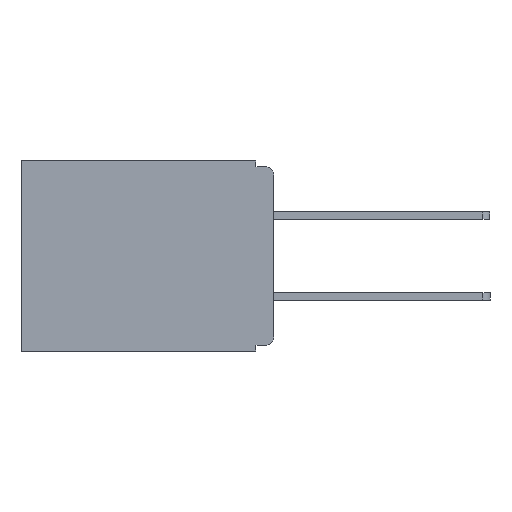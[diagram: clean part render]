
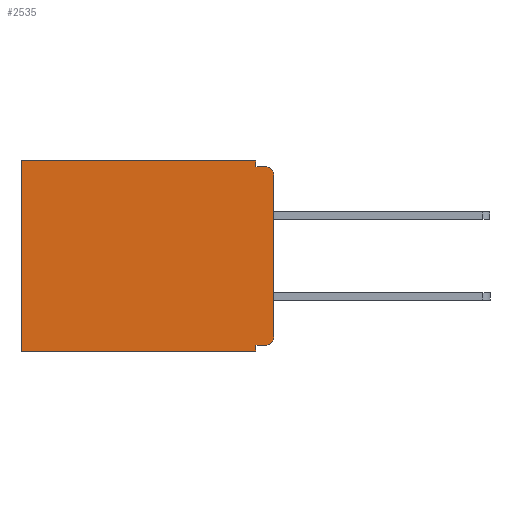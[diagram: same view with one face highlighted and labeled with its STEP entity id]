
A CAD part, left-side view. The second image highlights one B-rep face of the part: STEP entity #2535.
In plain terms, the highlighted planar face has unit normal (-1, 0, 0).
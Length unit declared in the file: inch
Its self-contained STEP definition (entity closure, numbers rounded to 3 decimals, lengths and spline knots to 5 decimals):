
#413 = ORIENTED_EDGE ( 'NONE', *, *, #1137, .T. ) ;
#1073 = DIRECTION ( 'NONE',  ( 1., 0., 0. ) ) ;
#1109 = DIRECTION ( 'NONE',  ( 0., 0., -1. ) ) ;
#1132 = PLANE ( 'NONE',  #11565 ) ;
#1137 = EDGE_CURVE ( 'NONE', #4834, #5431, #10066, .T. ) ;
#1713 = EDGE_CURVE ( 'NONE', #15782, #9134, #15542, .T. ) ;
#1774 = AXIS2_PLACEMENT_3D ( 'NONE', #14150, #14082, #16078 ) ;
#1932 = EDGE_CURVE ( 'NONE', #13408, #7439, #9005, .T. ) ;
#1935 = ORIENTED_EDGE ( 'NONE', *, *, #7380, .F. ) ;
#2269 = FACE_OUTER_BOUND ( 'NONE', #6078, .T. ) ;
#2293 = LINE ( 'NONE', #7403, #15918 ) ;
#2380 = ORIENTED_EDGE ( 'NONE', *, *, #4216, .F. ) ;
#2535 = ADVANCED_FACE ( 'NONE', ( #2269 ), #1132, .F. ) ;
#2682 = CARTESIAN_POINT ( 'NONE',  ( 0.3, 0.031, 0. ) ) ;
#3241 = EDGE_CURVE ( 'NONE', #10888, #13408, #11963, .T. ) ;
#4011 = LINE ( 'NONE', #2682, #7269 ) ;
#4216 = EDGE_CURVE ( 'NONE', #4271, #15782, #4011, .T. ) ;
#4271 = VERTEX_POINT ( 'NONE', #10977 ) ;
#4834 = VERTEX_POINT ( 'NONE', #14305 ) ;
#5072 = EDGE_CURVE ( 'NONE', #9587, #7439, #12307, .T. ) ;
#5298 = VECTOR ( 'NONE', #8970, 39.37008 ) ;
#5418 = VECTOR ( 'NONE', #11537, 39.37008 ) ;
#5431 = VERTEX_POINT ( 'NONE', #10803 ) ;
#5956 = CARTESIAN_POINT ( 'NONE',  ( 0.3, 0.437, -0.33 ) ) ;
#6078 = EDGE_LOOP ( 'NONE', ( #1935, #9300, #16006, #2380, #6184, #10108, #16790, #10494, #13841, #413 ) ) ;
#6184 = ORIENTED_EDGE ( 'NONE', *, *, #15045, .T. ) ;
#6335 = VERTEX_POINT ( 'NONE', #13143 ) ;
#6821 = EDGE_CURVE ( 'NONE', #6335, #9134, #17158, .T. ) ;
#6931 = DIRECTION ( 'NONE',  ( 0., 1., 0. ) ) ;
#6999 = DIRECTION ( 'NONE',  ( 0., 0., -1. ) ) ;
#7269 = VECTOR ( 'NONE', #10260, 39.37008 ) ;
#7380 = EDGE_CURVE ( 'NONE', #6335, #5431, #9245, .T. ) ;
#7403 = CARTESIAN_POINT ( 'NONE',  ( 0.3, 0., -0.32 ) ) ;
#7439 = VERTEX_POINT ( 'NONE', #5956 ) ;
#7558 = DIRECTION ( 'NONE',  ( 0., 0., -1. ) ) ;
#7664 = CARTESIAN_POINT ( 'NONE',  ( 0.3, 0., -0.33 ) ) ;
#7794 = CARTESIAN_POINT ( 'NONE',  ( 0.3, 0.437, -0.33 ) ) ;
#8663 = VECTOR ( 'NONE', #7558, 39.37008 ) ;
#8970 = DIRECTION ( 'NONE',  ( 0., 0., -1. ) ) ;
#9005 = LINE ( 'NONE', #14674, #5418 ) ;
#9134 = VERTEX_POINT ( 'NONE', #9169 ) ;
#9169 = CARTESIAN_POINT ( 'NONE',  ( 0.3, 0.015, -0.01 ) ) ;
#9245 = LINE ( 'NONE', #7664, #8663 ) ;
#9300 = ORIENTED_EDGE ( 'NONE', *, *, #6821, .T. ) ;
#9587 = VERTEX_POINT ( 'NONE', #12559 ) ;
#10066 = CIRCLE ( 'NONE', #1774, 0.015 ) ;
#10108 = ORIENTED_EDGE ( 'NONE', *, *, #5072, .T. ) ;
#10260 = DIRECTION ( 'NONE',  ( 0., 0., -1. ) ) ;
#10327 = EDGE_CURVE ( 'NONE', #4834, #10888, #2293, .T. ) ;
#10494 = ORIENTED_EDGE ( 'NONE', *, *, #3241, .F. ) ;
#10803 = CARTESIAN_POINT ( 'NONE',  ( 0.3, 0., -0.305 ) ) ;
#10888 = VERTEX_POINT ( 'NONE', #16247 ) ;
#10977 = CARTESIAN_POINT ( 'NONE',  ( 0.3, 0.031, 0. ) ) ;
#10994 = AXIS2_PLACEMENT_3D ( 'NONE', #16998, #16992, #16958 ) ;
#11537 = DIRECTION ( 'NONE',  ( 0., 1., 0. ) ) ;
#11551 = VECTOR ( 'NONE', #6999, 39.37008 ) ;
#11565 = AXIS2_PLACEMENT_3D ( 'NONE', #11581, #1073, #1109 ) ;
#11581 = CARTESIAN_POINT ( 'NONE',  ( 0.3, 0., -0.33 ) ) ;
#11963 = LINE ( 'NONE', #17038, #11551 ) ;
#12228 = VECTOR ( 'NONE', #13439, 39.37008 ) ;
#12297 = CARTESIAN_POINT ( 'NONE',  ( 0.3, 0.031, -0.01 ) ) ;
#12307 = LINE ( 'NONE', #7794, #5298 ) ;
#12559 = CARTESIAN_POINT ( 'NONE',  ( 0.3, 0.437, 0. ) ) ;
#13143 = CARTESIAN_POINT ( 'NONE',  ( 0.3, 0., -0.025 ) ) ;
#13408 = VERTEX_POINT ( 'NONE', #16879 ) ;
#13436 = CARTESIAN_POINT ( 'NONE',  ( 0.3, 0., -0.01 ) ) ;
#13439 = DIRECTION ( 'NONE',  ( 0., -1., 0. ) ) ;
#13504 = LINE ( 'NONE', #15857, #15666 ) ;
#13841 = ORIENTED_EDGE ( 'NONE', *, *, #10327, .F. ) ;
#14082 = DIRECTION ( 'NONE',  ( -1., 0., 0. ) ) ;
#14150 = CARTESIAN_POINT ( 'NONE',  ( 0.3, 0.015, -0.305 ) ) ;
#14305 = CARTESIAN_POINT ( 'NONE',  ( 0.3, 0.015, -0.32 ) ) ;
#14674 = CARTESIAN_POINT ( 'NONE',  ( 0.3, 0., -0.33 ) ) ;
#15045 = EDGE_CURVE ( 'NONE', #4271, #9587, #13504, .T. ) ;
#15061 = DIRECTION ( 'NONE',  ( 0., 1., 0. ) ) ;
#15542 = LINE ( 'NONE', #13436, #12228 ) ;
#15666 = VECTOR ( 'NONE', #6931, 39.37008 ) ;
#15782 = VERTEX_POINT ( 'NONE', #12297 ) ;
#15857 = CARTESIAN_POINT ( 'NONE',  ( 0.3, 0., 0. ) ) ;
#15918 = VECTOR ( 'NONE', #15061, 39.37008 ) ;
#16006 = ORIENTED_EDGE ( 'NONE', *, *, #1713, .F. ) ;
#16078 = DIRECTION ( 'NONE',  ( 0., 0., -1. ) ) ;
#16247 = CARTESIAN_POINT ( 'NONE',  ( 0.3, 0.031, -0.32 ) ) ;
#16790 = ORIENTED_EDGE ( 'NONE', *, *, #1932, .F. ) ;
#16879 = CARTESIAN_POINT ( 'NONE',  ( 0.3, 0.031, -0.33 ) ) ;
#16958 = DIRECTION ( 'NONE',  ( 0., 0., -1. ) ) ;
#16992 = DIRECTION ( 'NONE',  ( -1., 0., 0. ) ) ;
#16998 = CARTESIAN_POINT ( 'NONE',  ( 0.3, 0.015, -0.025 ) ) ;
#17038 = CARTESIAN_POINT ( 'NONE',  ( 0.3, 0.031, -0.33 ) ) ;
#17158 = CIRCLE ( 'NONE', #10994, 0.015 ) ;
